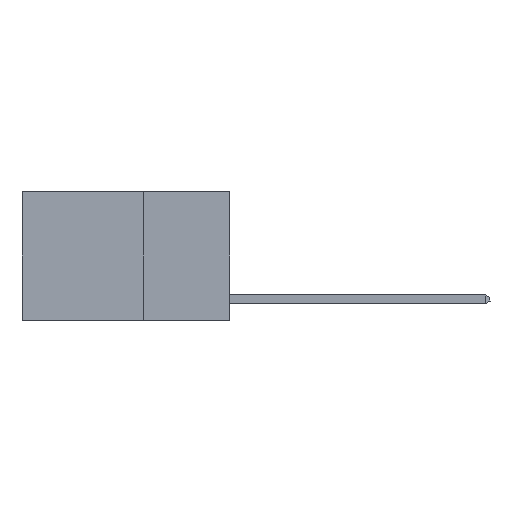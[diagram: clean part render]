
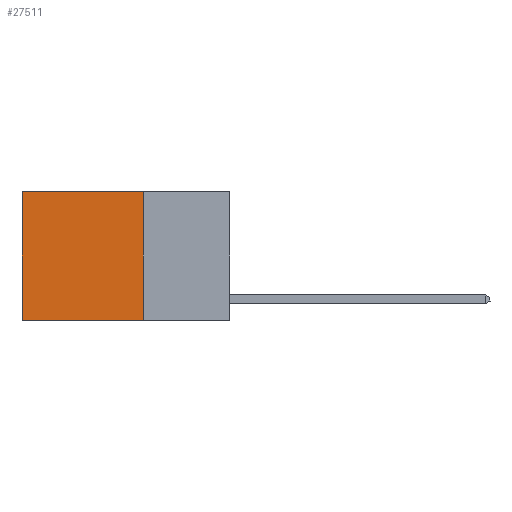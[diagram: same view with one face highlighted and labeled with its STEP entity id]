
A CAD part, left-side view. The second image highlights one B-rep face of the part: STEP entity #27511.
In plain terms, the highlighted planar face has unit normal (-1, 0, 0).
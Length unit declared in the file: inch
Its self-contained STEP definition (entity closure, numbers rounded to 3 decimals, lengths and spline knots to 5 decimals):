
#372 = LINE ( 'NONE', #22549, #12837 ) ;
#983 = CARTESIAN_POINT ( 'NONE',  ( 0.2625, 0.25, -0.37 ) ) ;
#1568 = DIRECTION ( 'NONE',  ( 0., 0., -1. ) ) ;
#3139 = VECTOR ( 'NONE', #15385, 39.37008 ) ;
#3330 = ORIENTED_EDGE ( 'NONE', *, *, #14582, .F. ) ;
#5090 = DIRECTION ( 'NONE',  ( 0., 0., -1. ) ) ;
#5943 = PLANE ( 'NONE',  #7303 ) ;
#6710 = ORIENTED_EDGE ( 'NONE', *, *, #13429, .T. ) ;
#7303 = AXIS2_PLACEMENT_3D ( 'NONE', #23484, #10153, #1568 ) ;
#7543 = LINE ( 'NONE', #11731, #24774 ) ;
#7789 = CARTESIAN_POINT ( 'NONE',  ( 0.2625, 0.25, 0. ) ) ;
#8500 = VECTOR ( 'NONE', #18928, 39.37008 ) ;
#8562 = EDGE_CURVE ( 'NONE', #17450, #16709, #372, .T. ) ;
#10153 = DIRECTION ( 'NONE',  ( 1., 0., 0. ) ) ;
#11465 = LINE ( 'NONE', #7789, #8500 ) ;
#11625 = DIRECTION ( 'NONE',  ( 0., 1., 0. ) ) ;
#11731 = CARTESIAN_POINT ( 'NONE',  ( 0.2625, 0.25, -0.37 ) ) ;
#12837 = VECTOR ( 'NONE', #5090, 39.37008 ) ;
#13141 = ORIENTED_EDGE ( 'NONE', *, *, #8562, .T. ) ;
#13429 = EDGE_CURVE ( 'NONE', #24280, #17450, #19394, .T. ) ;
#14582 = EDGE_CURVE ( 'NONE', #24280, #23592, #11465, .T. ) ;
#15069 = ORIENTED_EDGE ( 'NONE', *, *, #20229, .F. ) ;
#15385 = DIRECTION ( 'NONE',  ( 0., 1., 0. ) ) ;
#16709 = VERTEX_POINT ( 'NONE', #21620 ) ;
#17450 = VERTEX_POINT ( 'NONE', #21602 ) ;
#17802 = CARTESIAN_POINT ( 'NONE',  ( 0.2625, 0.25, 0. ) ) ;
#18928 = DIRECTION ( 'NONE',  ( 0., 0., -1. ) ) ;
#19394 = LINE ( 'NONE', #17802, #3139 ) ;
#20229 = EDGE_CURVE ( 'NONE', #23592, #16709, #7543, .T. ) ;
#20331 = EDGE_LOOP ( 'NONE', ( #13141, #15069, #3330, #6710 ) ) ;
#21602 = CARTESIAN_POINT ( 'NONE',  ( 0.2625, 0.6, 0. ) ) ;
#21620 = CARTESIAN_POINT ( 'NONE',  ( 0.2625, 0.6, -0.37 ) ) ;
#22549 = CARTESIAN_POINT ( 'NONE',  ( 0.2625, 0.6, 0. ) ) ;
#23365 = FACE_OUTER_BOUND ( 'NONE', #20331, .T. ) ;
#23484 = CARTESIAN_POINT ( 'NONE',  ( 0.2625, 0.25, 0. ) ) ;
#23592 = VERTEX_POINT ( 'NONE', #983 ) ;
#23978 = CARTESIAN_POINT ( 'NONE',  ( 0.2625, 0.25, 0. ) ) ;
#24280 = VERTEX_POINT ( 'NONE', #23978 ) ;
#24774 = VECTOR ( 'NONE', #11625, 39.37008 ) ;
#27511 = ADVANCED_FACE ( 'NONE', ( #23365 ), #5943, .F. ) ;
